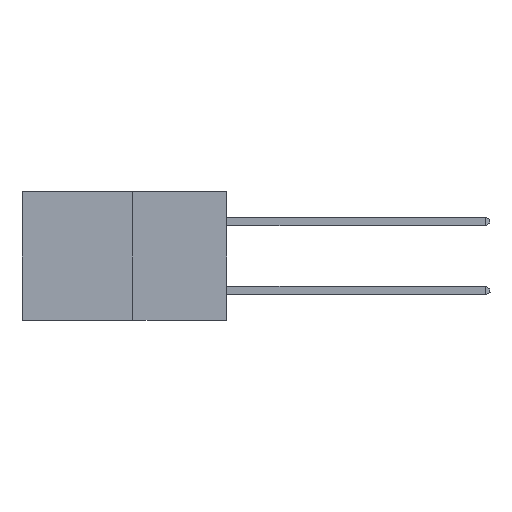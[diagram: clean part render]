
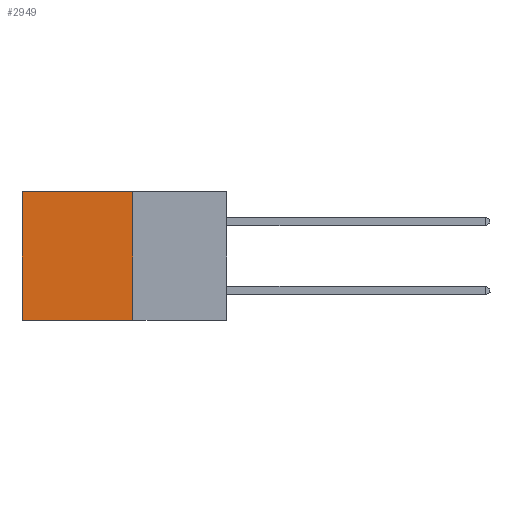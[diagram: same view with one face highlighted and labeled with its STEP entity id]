
A CAD part, left-side view. The second image highlights one B-rep face of the part: STEP entity #2949.
In plain terms, the highlighted planar face has unit normal (-1, 0, 0).
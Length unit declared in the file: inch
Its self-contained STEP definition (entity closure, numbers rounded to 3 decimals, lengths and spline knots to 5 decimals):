
#1010 = DIRECTION ( 'NONE',  ( 0., 1., 0. ) ) ;
#2258 = DIRECTION ( 'NONE',  ( 0., 0., -1. ) ) ;
#2359 = CARTESIAN_POINT ( 'NONE',  ( 0.277, 0.59, 0. ) ) ;
#2949 = ADVANCED_FACE ( 'NONE', ( #15905 ), #4826, .F. ) ;
#4826 = PLANE ( 'NONE',  #13964 ) ;
#4894 = CARTESIAN_POINT ( 'NONE',  ( 0.277, 0.27, -0.37 ) ) ;
#6127 = CARTESIAN_POINT ( 'NONE',  ( 0.277, 0.27, 0. ) ) ;
#6572 = VERTEX_POINT ( 'NONE', #9650 ) ;
#7169 = EDGE_LOOP ( 'NONE', ( #14661, #14897, #10173, #7765 ) ) ;
#7765 = ORIENTED_EDGE ( 'NONE', *, *, #14363, .T. ) ;
#7853 = LINE ( 'NONE', #14409, #22806 ) ;
#9650 = CARTESIAN_POINT ( 'NONE',  ( 0.277, 0.27, -0.37 ) ) ;
#10053 = EDGE_CURVE ( 'NONE', #12687, #6572, #22880, .T. ) ;
#10173 = ORIENTED_EDGE ( 'NONE', *, *, #10053, .F. ) ;
#11920 = VECTOR ( 'NONE', #21823, 39.37008 ) ;
#12687 = VERTEX_POINT ( 'NONE', #6127 ) ;
#12708 = LINE ( 'NONE', #12756, #17912 ) ;
#12741 = VERTEX_POINT ( 'NONE', #2359 ) ;
#12756 = CARTESIAN_POINT ( 'NONE',  ( 0.277, 0.27, 0. ) ) ;
#13964 = AXIS2_PLACEMENT_3D ( 'NONE', #4894, #21460, #2258 ) ;
#14363 = EDGE_CURVE ( 'NONE', #12687, #12741, #12708, .T. ) ;
#14409 = CARTESIAN_POINT ( 'NONE',  ( 0.277, 0.27, -0.37 ) ) ;
#14661 = ORIENTED_EDGE ( 'NONE', *, *, #17616, .T. ) ;
#14897 = ORIENTED_EDGE ( 'NONE', *, *, #18616, .F. ) ;
#15905 = FACE_OUTER_BOUND ( 'NONE', #7169, .T. ) ;
#15930 = VECTOR ( 'NONE', #20940, 39.37008 ) ;
#16525 = LINE ( 'NONE', #17118, #15930 ) ;
#17118 = CARTESIAN_POINT ( 'NONE',  ( 0.277, 0.59, -0.37 ) ) ;
#17616 = EDGE_CURVE ( 'NONE', #12741, #22020, #16525, .T. ) ;
#17912 = VECTOR ( 'NONE', #1010, 39.37008 ) ;
#18616 = EDGE_CURVE ( 'NONE', #6572, #22020, #7853, .T. ) ;
#20940 = DIRECTION ( 'NONE',  ( 0., 0., -1. ) ) ;
#21460 = DIRECTION ( 'NONE',  ( 1., 0., 0. ) ) ;
#21823 = DIRECTION ( 'NONE',  ( 0., 0., -1. ) ) ;
#21899 = CARTESIAN_POINT ( 'NONE',  ( 0.277, 0.27, -0.37 ) ) ;
#22020 = VERTEX_POINT ( 'NONE', #23202 ) ;
#22806 = VECTOR ( 'NONE', #24087, 39.37008 ) ;
#22880 = LINE ( 'NONE', #21899, #11920 ) ;
#23202 = CARTESIAN_POINT ( 'NONE',  ( 0.277, 0.59, -0.37 ) ) ;
#24087 = DIRECTION ( 'NONE',  ( 0., 1., 0. ) ) ;
